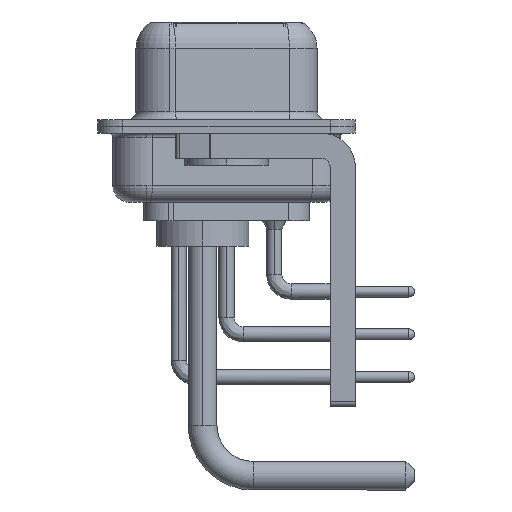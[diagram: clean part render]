
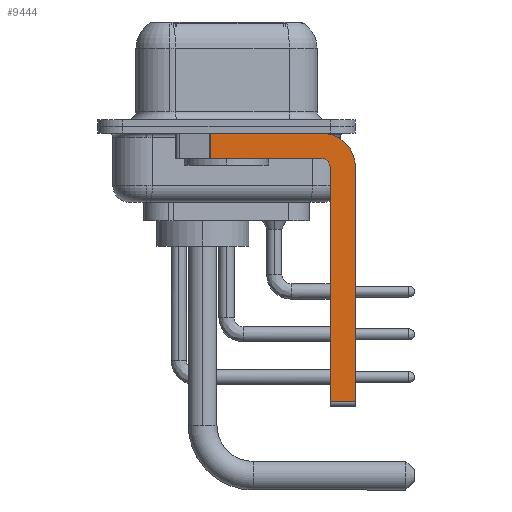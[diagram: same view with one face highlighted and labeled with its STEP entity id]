
A CAD part, left-side view. The second image highlights one B-rep face of the part: STEP entity #9444.
In plain terms, the highlighted planar face has unit normal (-1, 0, 0).
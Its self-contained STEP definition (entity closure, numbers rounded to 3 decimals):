
#448 = DIRECTION ( 'NONE',  ( 0., -1., 0. ) ) ;
#2477 = DIRECTION ( 'NONE',  ( 0., 0., -1. ) ) ;
#2503 = EDGE_CURVE ( 'NONE', #10840, #22217, #21607, .T. ) ;
#2762 = CARTESIAN_POINT ( 'NONE',  ( -2.9, -5.65, -2.4 ) ) ;
#3143 = ORIENTED_EDGE ( 'NONE', *, *, #2503, .T. ) ;
#3829 = DIRECTION ( 'NONE',  ( 0., 0., -1. ) ) ;
#4138 = EDGE_LOOP ( 'NONE', ( #9047, #16532, #6948, #17887, #22551, #3143, #20277, #5175 ) ) ;
#4269 = CARTESIAN_POINT ( 'NONE',  ( -2.9, -5.65, -0.4 ) ) ;
#4433 = AXIS2_PLACEMENT_3D ( 'NONE', #18776, #4935, #16357 ) ;
#4561 = VERTEX_POINT ( 'NONE', #19414 ) ;
#4935 = DIRECTION ( 'NONE',  ( -1., 0., 0. ) ) ;
#5175 = ORIENTED_EDGE ( 'NONE', *, *, #21930, .F. ) ;
#5212 = CARTESIAN_POINT ( 'NONE',  ( -2.9, -6.15, -16.35 ) ) ;
#5433 = CARTESIAN_POINT ( 'NONE',  ( -2.9, -6.15, -2.4 ) ) ;
#5446 = VECTOR ( 'NONE', #448, 1000. ) ;
#6329 = LINE ( 'NONE', #7908, #8532 ) ;
#6948 = ORIENTED_EDGE ( 'NONE', *, *, #23570, .F. ) ;
#7806 = CIRCLE ( 'NONE', #4433, 0.5 ) ;
#7908 = CARTESIAN_POINT ( 'NONE',  ( -2.9, -7.65, -2.4 ) ) ;
#8402 = CARTESIAN_POINT ( 'NONE',  ( -2.9, 3., -0.4 ) ) ;
#8532 = VECTOR ( 'NONE', #22057, 1000. ) ;
#9047 = ORIENTED_EDGE ( 'NONE', *, *, #14755, .F. ) ;
#9198 = VERTEX_POINT ( 'NONE', #17433 ) ;
#9435 = AXIS2_PLACEMENT_3D ( 'NONE', #21872, #12275, #9536 ) ;
#9444 = ADVANCED_FACE ( 'NONE', ( #11624 ), #14212, .F. ) ;
#9536 = DIRECTION ( 'NONE',  ( 0., 0., -1. ) ) ;
#9661 = AXIS2_PLACEMENT_3D ( 'NONE', #2762, #21519, #2477 ) ;
#10688 = VERTEX_POINT ( 'NONE', #13607 ) ;
#10840 = VERTEX_POINT ( 'NONE', #5212 ) ;
#10861 = DIRECTION ( 'NONE',  ( 0., 1., 0. ) ) ;
#11624 = FACE_OUTER_BOUND ( 'NONE', #4138, .T. ) ;
#11649 = CARTESIAN_POINT ( 'NONE',  ( -2.9, -7.65, -16.35 ) ) ;
#11668 = VERTEX_POINT ( 'NONE', #24894 ) ;
#12275 = DIRECTION ( 'NONE',  ( 1., 0., 0. ) ) ;
#12693 = LINE ( 'NONE', #15299, #25125 ) ;
#12954 = CARTESIAN_POINT ( 'NONE',  ( -2.9, 0.978, -1.9 ) ) ;
#13607 = CARTESIAN_POINT ( 'NONE',  ( -2.9, -7.65, -2.4 ) ) ;
#13609 = EDGE_CURVE ( 'NONE', #11668, #4561, #26686, .T. ) ;
#14212 = PLANE ( 'NONE',  #9661 ) ;
#14755 = EDGE_CURVE ( 'NONE', #11668, #17779, #15725, .T. ) ;
#15299 = CARTESIAN_POINT ( 'NONE',  ( -2.9, -5.65, -1.9 ) ) ;
#15725 = LINE ( 'NONE', #8402, #19760 ) ;
#16357 = DIRECTION ( 'NONE',  ( 0., 0., 1. ) ) ;
#16532 = ORIENTED_EDGE ( 'NONE', *, *, #13609, .T. ) ;
#16641 = EDGE_CURVE ( 'NONE', #10840, #24021, #23994, .T. ) ;
#17433 = CARTESIAN_POINT ( 'NONE',  ( -2.9, -5.65, -1.9 ) ) ;
#17697 = DIRECTION ( 'NONE',  ( 0., -1., 0. ) ) ;
#17779 = VERTEX_POINT ( 'NONE', #4269 ) ;
#17887 = ORIENTED_EDGE ( 'NONE', *, *, #19743, .F. ) ;
#18260 = VECTOR ( 'NONE', #3829, 1000. ) ;
#18776 = CARTESIAN_POINT ( 'NONE',  ( -2.9, -5.65, -2.4 ) ) ;
#18893 = VECTOR ( 'NONE', #19891, 1000. ) ;
#19414 = CARTESIAN_POINT ( 'NONE',  ( -2.9, 0.978, -1.9 ) ) ;
#19743 = EDGE_CURVE ( 'NONE', #24021, #9198, #7806, .T. ) ;
#19760 = VECTOR ( 'NONE', #17697, 1000. ) ;
#19891 = DIRECTION ( 'NONE',  ( 0., 0., 1. ) ) ;
#20277 = ORIENTED_EDGE ( 'NONE', *, *, #23162, .F. ) ;
#20660 = CIRCLE ( 'NONE', #9435, 2. ) ;
#21163 = CARTESIAN_POINT ( 'NONE',  ( -2.9, -5.65, -16.35 ) ) ;
#21519 = DIRECTION ( 'NONE',  ( 1., 0., 0. ) ) ;
#21607 = LINE ( 'NONE', #21163, #5446 ) ;
#21872 = CARTESIAN_POINT ( 'NONE',  ( -2.9, -5.65, -2.4 ) ) ;
#21930 = EDGE_CURVE ( 'NONE', #17779, #10688, #20660, .T. ) ;
#22057 = DIRECTION ( 'NONE',  ( 0., 0., -1. ) ) ;
#22217 = VERTEX_POINT ( 'NONE', #11649 ) ;
#22551 = ORIENTED_EDGE ( 'NONE', *, *, #16641, .F. ) ;
#23162 = EDGE_CURVE ( 'NONE', #10688, #22217, #6329, .T. ) ;
#23570 = EDGE_CURVE ( 'NONE', #9198, #4561, #12693, .T. ) ;
#23994 = LINE ( 'NONE', #28875, #18893 ) ;
#24021 = VERTEX_POINT ( 'NONE', #5433 ) ;
#24894 = CARTESIAN_POINT ( 'NONE',  ( -2.9, 0.978, -0.4 ) ) ;
#25125 = VECTOR ( 'NONE', #10861, 1000. ) ;
#26686 = LINE ( 'NONE', #12954, #18260 ) ;
#28875 = CARTESIAN_POINT ( 'NONE',  ( -2.9, -6.15, -16.6 ) ) ;
